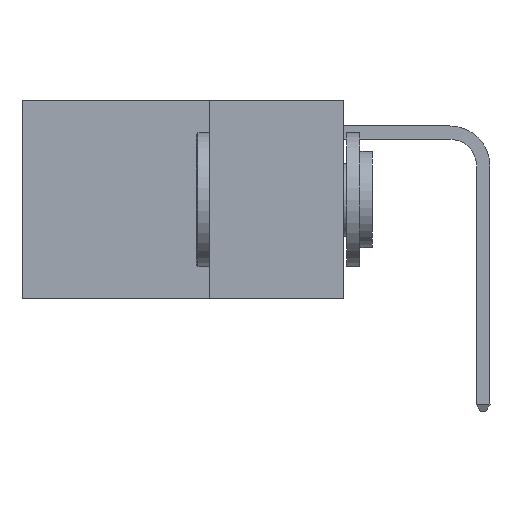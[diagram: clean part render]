
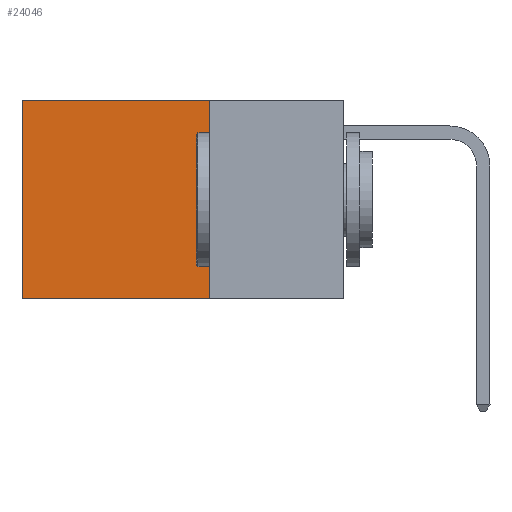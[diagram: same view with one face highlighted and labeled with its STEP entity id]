
A CAD part, left-side view. The second image highlights one B-rep face of the part: STEP entity #24046.
In plain terms, the highlighted planar face has unit normal (-1, 0, 0).
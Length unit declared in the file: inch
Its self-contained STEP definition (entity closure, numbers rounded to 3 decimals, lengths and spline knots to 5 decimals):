
#609 = CARTESIAN_POINT ( 'NONE',  ( 0.2625, 0.6, -0.37 ) ) ;
#2442 = CARTESIAN_POINT ( 'NONE',  ( 0.2625, 0.25, 0. ) ) ;
#2448 = VECTOR ( 'NONE', #9342, 39.37008 ) ;
#3933 = DIRECTION ( 'NONE',  ( 1., 0., 0. ) ) ;
#4290 = CARTESIAN_POINT ( 'NONE',  ( 0.2625, 0.25, 0. ) ) ;
#4494 = LINE ( 'NONE', #23953, #9567 ) ;
#4779 = VERTEX_POINT ( 'NONE', #609 ) ;
#5575 = EDGE_CURVE ( 'NONE', #18316, #4779, #4494, .T. ) ;
#6389 = LINE ( 'NONE', #2442, #25127 ) ;
#6630 = CARTESIAN_POINT ( 'NONE',  ( 0.2625, 0.25, -0.37 ) ) ;
#7423 = LINE ( 'NONE', #13044, #2448 ) ;
#7764 = EDGE_LOOP ( 'NONE', ( #11931, #18982, #8458, #18872 ) ) ;
#8013 = CARTESIAN_POINT ( 'NONE',  ( 0.2625, 0.25, 0. ) ) ;
#8315 = LINE ( 'NONE', #20227, #15369 ) ;
#8458 = ORIENTED_EDGE ( 'NONE', *, *, #25044, .F. ) ;
#9342 = DIRECTION ( 'NONE',  ( 0., 0., -1. ) ) ;
#9567 = VECTOR ( 'NONE', #12511, 39.37008 ) ;
#11931 = ORIENTED_EDGE ( 'NONE', *, *, #18035, .T. ) ;
#11939 = DIRECTION ( 'NONE',  ( 0., 0., -1. ) ) ;
#12511 = DIRECTION ( 'NONE',  ( 0., 1., 0. ) ) ;
#13044 = CARTESIAN_POINT ( 'NONE',  ( 0.2625, 0.6, 0. ) ) ;
#13807 = DIRECTION ( 'NONE',  ( 0., 1., 0. ) ) ;
#15369 = VECTOR ( 'NONE', #24194, 39.37008 ) ;
#15901 = CARTESIAN_POINT ( 'NONE',  ( 0.2625, 0.6, 0. ) ) ;
#17797 = AXIS2_PLACEMENT_3D ( 'NONE', #8013, #3933, #11939 ) ;
#18035 = EDGE_CURVE ( 'NONE', #21349, #4779, #7423, .T. ) ;
#18316 = VERTEX_POINT ( 'NONE', #6630 ) ;
#18872 = ORIENTED_EDGE ( 'NONE', *, *, #23129, .T. ) ;
#18982 = ORIENTED_EDGE ( 'NONE', *, *, #5575, .F. ) ;
#19648 = FACE_OUTER_BOUND ( 'NONE', #7764, .T. ) ;
#20227 = CARTESIAN_POINT ( 'NONE',  ( 0.2625, 0.25, 0. ) ) ;
#21349 = VERTEX_POINT ( 'NONE', #15901 ) ;
#21442 = PLANE ( 'NONE',  #17797 ) ;
#23129 = EDGE_CURVE ( 'NONE', #23284, #21349, #6389, .T. ) ;
#23284 = VERTEX_POINT ( 'NONE', #4290 ) ;
#23953 = CARTESIAN_POINT ( 'NONE',  ( 0.2625, 0.25, -0.37 ) ) ;
#24046 = ADVANCED_FACE ( 'NONE', ( #19648 ), #21442, .F. ) ;
#24194 = DIRECTION ( 'NONE',  ( 0., 0., -1. ) ) ;
#25044 = EDGE_CURVE ( 'NONE', #23284, #18316, #8315, .T. ) ;
#25127 = VECTOR ( 'NONE', #13807, 39.37008 ) ;
